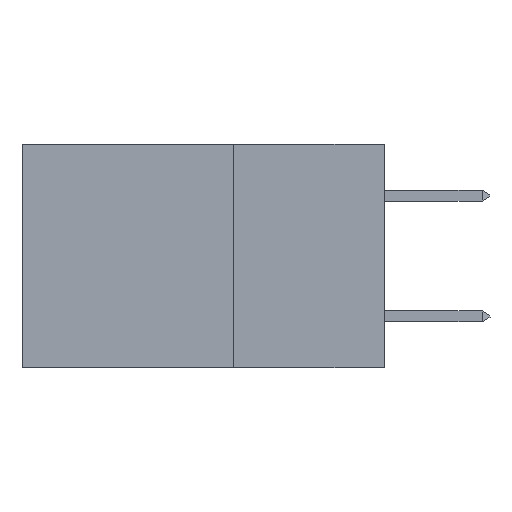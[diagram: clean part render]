
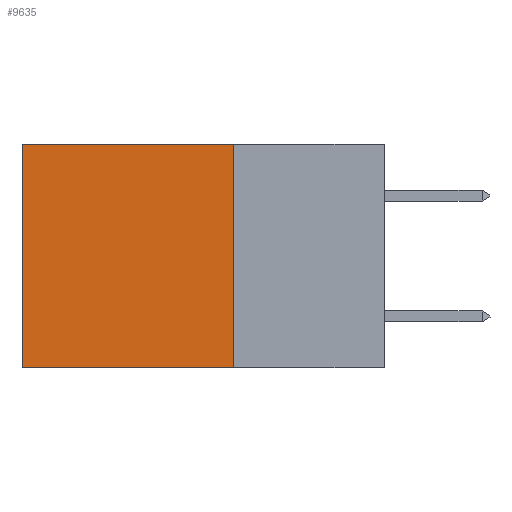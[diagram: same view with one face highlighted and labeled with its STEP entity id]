
A CAD part, left-side view. The second image highlights one B-rep face of the part: STEP entity #9635.
In plain terms, the highlighted planar face has unit normal (-1, 0, 0).
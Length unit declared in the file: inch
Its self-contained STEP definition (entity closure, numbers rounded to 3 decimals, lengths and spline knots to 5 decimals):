
#818 = CARTESIAN_POINT ( 'NONE',  ( 0.2875, 0.25, -0.37 ) ) ;
#949 = VERTEX_POINT ( 'NONE', #12175 ) ;
#1356 = ORIENTED_EDGE ( 'NONE', *, *, #8262, .T. ) ;
#1627 = VERTEX_POINT ( 'NONE', #19351 ) ;
#2624 = CARTESIAN_POINT ( 'NONE',  ( 0.2875, 0.25, -0.37 ) ) ;
#3340 = DIRECTION ( 'NONE',  ( 0., 1., 0. ) ) ;
#3487 = EDGE_CURVE ( 'NONE', #949, #9716, #14593, .T. ) ;
#4291 = PLANE ( 'NONE',  #16325 ) ;
#5142 = CARTESIAN_POINT ( 'NONE',  ( 0.2875, 0.25, 0. ) ) ;
#7421 = FACE_OUTER_BOUND ( 'NONE', #9619, .T. ) ;
#7593 = ORIENTED_EDGE ( 'NONE', *, *, #18919, .F. ) ;
#8083 = ORIENTED_EDGE ( 'NONE', *, *, #3487, .F. ) ;
#8262 = EDGE_CURVE ( 'NONE', #949, #1627, #10201, .T. ) ;
#8604 = CARTESIAN_POINT ( 'NONE',  ( 0.2875, 0.25, 0. ) ) ;
#9379 = LINE ( 'NONE', #2624, #13583 ) ;
#9619 = EDGE_LOOP ( 'NONE', ( #16246, #7593, #8083, #1356 ) ) ;
#9635 = ADVANCED_FACE ( 'NONE', ( #7421 ), #4291, .F. ) ;
#9645 = DIRECTION ( 'NONE',  ( 1., 0., 0. ) ) ;
#9673 = VECTOR ( 'NONE', #3340, 39.37008 ) ;
#9716 = VERTEX_POINT ( 'NONE', #818 ) ;
#10201 = LINE ( 'NONE', #5142, #9673 ) ;
#10299 = VECTOR ( 'NONE', #20977, 39.37008 ) ;
#10494 = CARTESIAN_POINT ( 'NONE',  ( 0.2875, 0.6, -0.37 ) ) ;
#10709 = CARTESIAN_POINT ( 'NONE',  ( 0.2875, 0.6, 0. ) ) ;
#11760 = VERTEX_POINT ( 'NONE', #10494 ) ;
#12175 = CARTESIAN_POINT ( 'NONE',  ( 0.2875, 0.25, 0. ) ) ;
#13583 = VECTOR ( 'NONE', #20401, 39.37008 ) ;
#14593 = LINE ( 'NONE', #8604, #10299 ) ;
#15186 = LINE ( 'NONE', #10709, #18222 ) ;
#15619 = EDGE_CURVE ( 'NONE', #1627, #11760, #15186, .T. ) ;
#16246 = ORIENTED_EDGE ( 'NONE', *, *, #15619, .T. ) ;
#16325 = AXIS2_PLACEMENT_3D ( 'NONE', #20280, #9645, #21972 ) ;
#18222 = VECTOR ( 'NONE', #19623, 39.37008 ) ;
#18919 = EDGE_CURVE ( 'NONE', #9716, #11760, #9379, .T. ) ;
#19351 = CARTESIAN_POINT ( 'NONE',  ( 0.2875, 0.6, 0. ) ) ;
#19623 = DIRECTION ( 'NONE',  ( 0., 0., -1. ) ) ;
#20280 = CARTESIAN_POINT ( 'NONE',  ( 0.2875, 0.25, 0. ) ) ;
#20401 = DIRECTION ( 'NONE',  ( 0., 1., 0. ) ) ;
#20977 = DIRECTION ( 'NONE',  ( 0., 0., -1. ) ) ;
#21972 = DIRECTION ( 'NONE',  ( 0., 0., -1. ) ) ;
